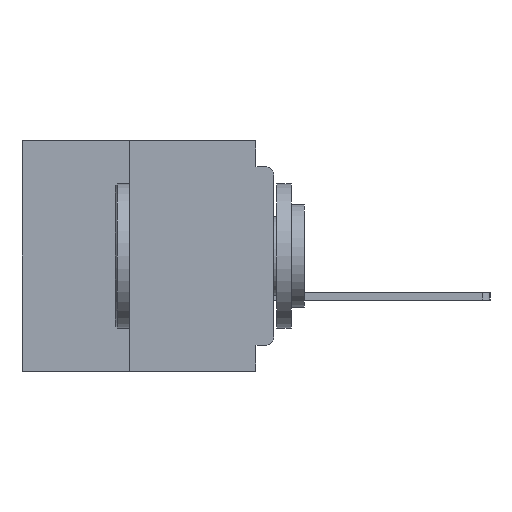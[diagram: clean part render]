
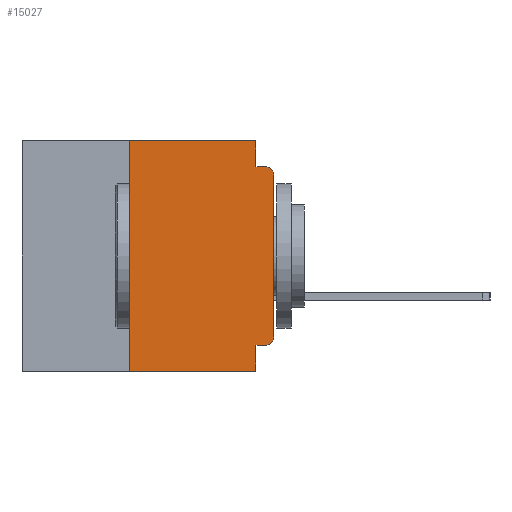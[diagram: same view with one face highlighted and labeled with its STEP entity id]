
A CAD part, left-side view. The second image highlights one B-rep face of the part: STEP entity #15027.
In plain terms, the highlighted planar face has unit normal (-1, 0, 0).
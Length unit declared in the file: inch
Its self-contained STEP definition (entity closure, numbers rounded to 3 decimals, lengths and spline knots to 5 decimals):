
#1989 = CARTESIAN_POINT ( 'NONE',  ( 0., 0.031, -0.4 ) ) ;
#3097 = LINE ( 'NONE', #31525, #52546 ) ;
#3582 = CIRCLE ( 'NONE', #35016, 0.015 ) ;
#3818 = VERTEX_POINT ( 'NONE', #49720 ) ;
#3928 = AXIS2_PLACEMENT_3D ( 'NONE', #16615, #50048, #21453 ) ;
#4676 = ORIENTED_EDGE ( 'NONE', *, *, #16348, .F. ) ;
#5231 = EDGE_CURVE ( 'NONE', #7501, #30713, #3097, .T. ) ;
#6511 = LINE ( 'NONE', #10502, #41854 ) ;
#7142 = CARTESIAN_POINT ( 'NONE',  ( 0., 0.437, 0. ) ) ;
#7501 = VERTEX_POINT ( 'NONE', #38858 ) ;
#8940 = EDGE_CURVE ( 'NONE', #57298, #30427, #29889, .T. ) ;
#10502 = CARTESIAN_POINT ( 'NONE',  ( 0., 0., -0.355 ) ) ;
#12003 = DIRECTION ( 'NONE',  ( 1., 0., 0. ) ) ;
#12431 = CARTESIAN_POINT ( 'NONE',  ( 0., 0.25, -0.4 ) ) ;
#12612 = CARTESIAN_POINT ( 'NONE',  ( 0., 0.015, -0.355 ) ) ;
#12734 = CARTESIAN_POINT ( 'NONE',  ( 0., 0.25, -0.4 ) ) ;
#13640 = CARTESIAN_POINT ( 'NONE',  ( 0., 0.015, -0.045 ) ) ;
#14531 = CARTESIAN_POINT ( 'NONE',  ( 0., 0.437, -0.4 ) ) ;
#15027 = ADVANCED_FACE ( 'NONE', ( #42534 ), #40751, .F. ) ;
#15071 = ORIENTED_EDGE ( 'NONE', *, *, #35501, .F. ) ;
#16101 = DIRECTION ( 'NONE',  ( -1., 0., 0. ) ) ;
#16230 = EDGE_CURVE ( 'NONE', #30713, #52564, #55135, .T. ) ;
#16348 = EDGE_CURVE ( 'NONE', #29340, #22263, #26889, .T. ) ;
#16549 = EDGE_CURVE ( 'NONE', #29340, #3818, #24584, .T. ) ;
#16615 = CARTESIAN_POINT ( 'NONE',  ( 0., 0.015, -0.34 ) ) ;
#16788 = VECTOR ( 'NONE', #43673, 39.37008 ) ;
#17496 = DIRECTION ( 'NONE',  ( 0., 0., 1. ) ) ;
#18311 = LINE ( 'NONE', #57699, #16788 ) ;
#19111 = EDGE_CURVE ( 'NONE', #22263, #7501, #18311, .T. ) ;
#19359 = DIRECTION ( 'NONE',  ( 0., -1., 0. ) ) ;
#21135 = EDGE_CURVE ( 'NONE', #23082, #57298, #55836, .T. ) ;
#21258 = DIRECTION ( 'NONE',  ( 0., 0., -1. ) ) ;
#21453 = DIRECTION ( 'NONE',  ( 0., 0., -1. ) ) ;
#22263 = VERTEX_POINT ( 'NONE', #53209 ) ;
#23082 = VERTEX_POINT ( 'NONE', #12612 ) ;
#24584 = LINE ( 'NONE', #14531, #48443 ) ;
#25184 = ORIENTED_EDGE ( 'NONE', *, *, #8940, .T. ) ;
#25320 = ORIENTED_EDGE ( 'NONE', *, *, #21135, .T. ) ;
#26889 = LINE ( 'NONE', #12431, #60254 ) ;
#28384 = VECTOR ( 'NONE', #58913, 39.37008 ) ;
#28579 = CARTESIAN_POINT ( 'NONE',  ( 0., 0.031, -0.045 ) ) ;
#29340 = VERTEX_POINT ( 'NONE', #12734 ) ;
#29889 = LINE ( 'NONE', #44898, #28384 ) ;
#30427 = VERTEX_POINT ( 'NONE', #45476 ) ;
#30713 = VERTEX_POINT ( 'NONE', #28579 ) ;
#31227 = ORIENTED_EDGE ( 'NONE', *, *, #5231, .F. ) ;
#31410 = VECTOR ( 'NONE', #54813, 39.37008 ) ;
#31525 = CARTESIAN_POINT ( 'NONE',  ( 0., 0.031, 0. ) ) ;
#31634 = ORIENTED_EDGE ( 'NONE', *, *, #16230, .F. ) ;
#31747 = DIRECTION ( 'NONE',  ( 0., 0., -1. ) ) ;
#34284 = ORIENTED_EDGE ( 'NONE', *, *, #19111, .F. ) ;
#34522 = DIRECTION ( 'NONE',  ( 0., 1., 0. ) ) ;
#35016 = AXIS2_PLACEMENT_3D ( 'NONE', #44781, #16101, #49521 ) ;
#35501 = EDGE_CURVE ( 'NONE', #23082, #46723, #6511, .T. ) ;
#35976 = CARTESIAN_POINT ( 'NONE',  ( 0., 0., -0.34 ) ) ;
#38858 = CARTESIAN_POINT ( 'NONE',  ( 0., 0.031, 0. ) ) ;
#39614 = LINE ( 'NONE', #1989, #61782 ) ;
#40567 = CARTESIAN_POINT ( 'NONE',  ( 0., 0., -0.045 ) ) ;
#40751 = PLANE ( 'NONE',  #53005 ) ;
#41854 = VECTOR ( 'NONE', #34522, 39.37008 ) ;
#42534 = FACE_OUTER_BOUND ( 'NONE', #47870, .T. ) ;
#43673 = DIRECTION ( 'NONE',  ( 0., -1., 0. ) ) ;
#44781 = CARTESIAN_POINT ( 'NONE',  ( 0., 0.015, -0.06 ) ) ;
#44898 = CARTESIAN_POINT ( 'NONE',  ( 0., 0., 0. ) ) ;
#45476 = CARTESIAN_POINT ( 'NONE',  ( 0., 0., -0.06 ) ) ;
#45516 = DIRECTION ( 'NONE',  ( 0., 0., -1. ) ) ;
#46723 = VERTEX_POINT ( 'NONE', #47447 ) ;
#47447 = CARTESIAN_POINT ( 'NONE',  ( 0., 0.031, -0.355 ) ) ;
#47870 = EDGE_LOOP ( 'NONE', ( #25184, #54552, #31634, #31227, #34284, #4676, #50513, #53038, #15071, #25320 ) ) ;
#48205 = EDGE_CURVE ( 'NONE', #30427, #52564, #3582, .T. ) ;
#48443 = VECTOR ( 'NONE', #19359, 39.37008 ) ;
#49521 = DIRECTION ( 'NONE',  ( 0., 0., -1. ) ) ;
#49720 = CARTESIAN_POINT ( 'NONE',  ( 0., 0.031, -0.4 ) ) ;
#50048 = DIRECTION ( 'NONE',  ( -1., 0., 0. ) ) ;
#50513 = ORIENTED_EDGE ( 'NONE', *, *, #16549, .T. ) ;
#52546 = VECTOR ( 'NONE', #31747, 39.37008 ) ;
#52564 = VERTEX_POINT ( 'NONE', #13640 ) ;
#53005 = AXIS2_PLACEMENT_3D ( 'NONE', #7142, #12003, #45516 ) ;
#53038 = ORIENTED_EDGE ( 'NONE', *, *, #55457, .F. ) ;
#53209 = CARTESIAN_POINT ( 'NONE',  ( 0., 0.25, 0. ) ) ;
#54552 = ORIENTED_EDGE ( 'NONE', *, *, #48205, .T. ) ;
#54813 = DIRECTION ( 'NONE',  ( 0., -1., 0. ) ) ;
#55135 = LINE ( 'NONE', #40567, #31410 ) ;
#55457 = EDGE_CURVE ( 'NONE', #46723, #3818, #39614, .T. ) ;
#55836 = CIRCLE ( 'NONE', #3928, 0.015 ) ;
#57298 = VERTEX_POINT ( 'NONE', #35976 ) ;
#57699 = CARTESIAN_POINT ( 'NONE',  ( 0., 0.437, 0. ) ) ;
#58913 = DIRECTION ( 'NONE',  ( 0., 0., 1. ) ) ;
#60254 = VECTOR ( 'NONE', #17496, 39.37008 ) ;
#61782 = VECTOR ( 'NONE', #21258, 39.37008 ) ;
